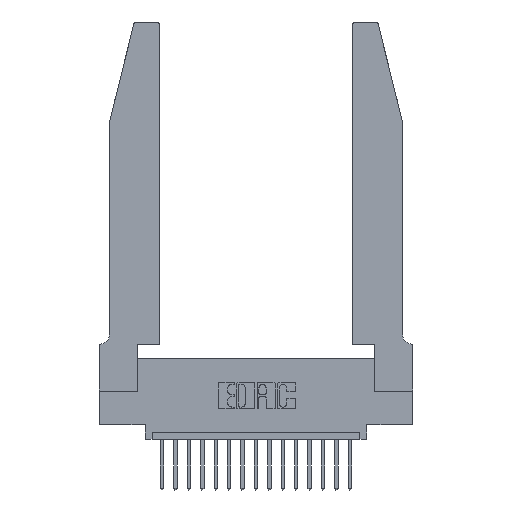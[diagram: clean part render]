
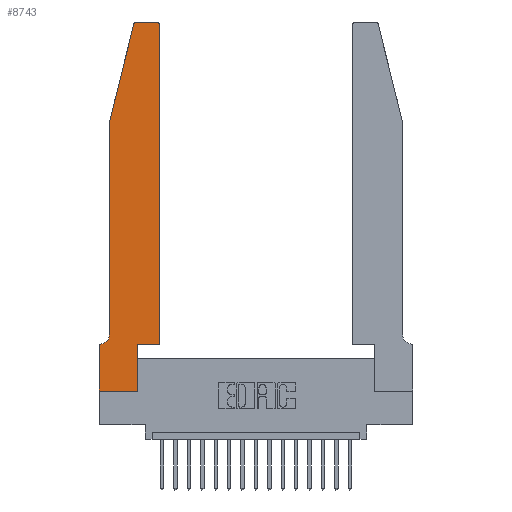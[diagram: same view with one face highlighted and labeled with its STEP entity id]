
A CAD part, top view. The second image highlights one B-rep face of the part: STEP entity #8743.
In plain terms, the highlighted planar face has unit normal (0, 0, 1).
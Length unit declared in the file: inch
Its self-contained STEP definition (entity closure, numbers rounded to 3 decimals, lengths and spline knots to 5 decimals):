
#88 = VECTOR ( 'NONE', #19407, 39.37008 ) ;
#260 = CIRCLE ( 'NONE', #11740, 0.03 ) ;
#834 = VERTEX_POINT ( 'NONE', #14219 ) ;
#893 = CIRCLE ( 'NONE', #18518, 0.03 ) ;
#983 = ORIENTED_EDGE ( 'NONE', *, *, #5429, .T. ) ;
#1018 = VECTOR ( 'NONE', #5534, 39.37008 ) ;
#1057 = FACE_OUTER_BOUND ( 'NONE', #17933, .T. ) ;
#1080 = VERTEX_POINT ( 'NONE', #16287 ) ;
#1220 = CARTESIAN_POINT ( 'NONE',  ( 0.0055, 0.42, 0.37 ) ) ;
#1270 = DIRECTION ( 'NONE',  ( 0., 1., 0. ) ) ;
#1604 = VERTEX_POINT ( 'NONE', #9121 ) ;
#2000 = EDGE_CURVE ( 'NONE', #5994, #1080, #260, .T. ) ;
#2140 = CARTESIAN_POINT ( 'NONE',  ( 0.25487, 2.72718, 0.37 ) ) ;
#2611 = LINE ( 'NONE', #16201, #7883 ) ;
#3807 = ORIENTED_EDGE ( 'NONE', *, *, #18203, .T. ) ;
#3827 = ORIENTED_EDGE ( 'NONE', *, *, #16820, .T. ) ;
#3977 = VERTEX_POINT ( 'NONE', #17043 ) ;
#4001 = VERTEX_POINT ( 'NONE', #5031 ) ;
#4025 = DIRECTION ( 'NONE',  ( 1., 0., 0. ) ) ;
#4074 = VERTEX_POINT ( 'NONE', #11245 ) ;
#4116 = LINE ( 'NONE', #8658, #88 ) ;
#4330 = LINE ( 'NONE', #9478, #1018 ) ;
#4439 = DIRECTION ( 'NONE',  ( -1., 0., 0. ) ) ;
#4830 = VERTEX_POINT ( 'NONE', #12099 ) ;
#5031 = CARTESIAN_POINT ( 'NONE',  ( 0.0055, 0.35, 0.37 ) ) ;
#5297 = VECTOR ( 'NONE', #4439, 39.37008 ) ;
#5429 = EDGE_CURVE ( 'NONE', #4074, #5994, #6590, .T. ) ;
#5534 = DIRECTION ( 'NONE',  ( 1., 0., 0. ) ) ;
#5660 = DIRECTION ( 'NONE',  ( -1., 0., 0. ) ) ;
#5920 = VECTOR ( 'NONE', #12808, 39.37008 ) ;
#5974 = EDGE_CURVE ( 'NONE', #13099, #4001, #12536, .T. ) ;
#5994 = VERTEX_POINT ( 'NONE', #8876 ) ;
#6364 = CARTESIAN_POINT ( 'NONE',  ( 0., 0., 0.37 ) ) ;
#6590 = LINE ( 'NONE', #9124, #18580 ) ;
#6973 = PLANE ( 'NONE',  #10101 ) ;
#7408 = VECTOR ( 'NONE', #11637, 39.37008 ) ;
#7510 = ORIENTED_EDGE ( 'NONE', *, *, #14543, .T. ) ;
#7883 = VECTOR ( 'NONE', #5660, 39.37008 ) ;
#7919 = CARTESIAN_POINT ( 'NONE',  ( 0.284, 2.72, 0.37 ) ) ;
#8313 = ORIENTED_EDGE ( 'NONE', *, *, #17639, .T. ) ;
#8387 = CARTESIAN_POINT ( 'NONE',  ( 0., 0.35, 0.37 ) ) ;
#8507 = DIRECTION ( 'NONE',  ( 0., 0., 1. ) ) ;
#8658 = CARTESIAN_POINT ( 'NONE',  ( 0.0755, 2., 0.37 ) ) ;
#8666 = CARTESIAN_POINT ( 'NONE',  ( 0.4505, 0.35, 0.37 ) ) ;
#8684 = VERTEX_POINT ( 'NONE', #2140 ) ;
#8743 = ADVANCED_FACE ( 'NONE', ( #1057 ), #6973, .T. ) ;
#8761 = LINE ( 'NONE', #11251, #5920 ) ;
#8876 = CARTESIAN_POINT ( 'NONE',  ( 0.4505, 2.72, 0.37 ) ) ;
#9121 = CARTESIAN_POINT ( 'NONE',  ( 0.2865, 0.35, 0.37 ) ) ;
#9124 = CARTESIAN_POINT ( 'NONE',  ( 0.4505, 0.35, 0.37 ) ) ;
#9411 = EDGE_CURVE ( 'NONE', #8684, #18680, #4116, .T. ) ;
#9478 = CARTESIAN_POINT ( 'NONE',  ( 0., 0., 0.37 ) ) ;
#9704 = LINE ( 'NONE', #6364, #10393 ) ;
#10101 = AXIS2_PLACEMENT_3D ( 'NONE', #8387, #8507, #17453 ) ;
#10141 = VERTEX_POINT ( 'NONE', #14768 ) ;
#10278 = AXIS2_PLACEMENT_3D ( 'NONE', #1220, #18346, #15186 ) ;
#10393 = VECTOR ( 'NONE', #18820, 39.37008 ) ;
#10521 = CARTESIAN_POINT ( 'NONE',  ( 0.0755, 0.35, 0.37 ) ) ;
#10523 = LINE ( 'NONE', #10521, #5297 ) ;
#10629 = CARTESIAN_POINT ( 'NONE',  ( 0.0755, 0.42, 0.37 ) ) ;
#11245 = CARTESIAN_POINT ( 'NONE',  ( 0.4505, 0.35, 0.37 ) ) ;
#11251 = CARTESIAN_POINT ( 'NONE',  ( 0.0755, 2., 0.37 ) ) ;
#11637 = DIRECTION ( 'NONE',  ( 0., 1., 0. ) ) ;
#11698 = CARTESIAN_POINT ( 'NONE',  ( 0.4205, 2.72, 0.37 ) ) ;
#11740 = AXIS2_PLACEMENT_3D ( 'NONE', #11698, #17776, #4025 ) ;
#12099 = CARTESIAN_POINT ( 'NONE',  ( 0.284, 2.75, 0.37 ) ) ;
#12390 = ORIENTED_EDGE ( 'NONE', *, *, #17186, .T. ) ;
#12536 = CIRCLE ( 'NONE', #10278, 0.07 ) ;
#12636 = ORIENTED_EDGE ( 'NONE', *, *, #9411, .T. ) ;
#12808 = DIRECTION ( 'NONE',  ( 0., -1., 0. ) ) ;
#13099 = VERTEX_POINT ( 'NONE', #10629 ) ;
#13935 = EDGE_CURVE ( 'NONE', #4830, #8684, #893, .T. ) ;
#14219 = CARTESIAN_POINT ( 'NONE',  ( 0., 0.35, 0.37 ) ) ;
#14221 = EDGE_CURVE ( 'NONE', #834, #3977, #9704, .T. ) ;
#14241 = ORIENTED_EDGE ( 'NONE', *, *, #19699, .T. ) ;
#14543 = EDGE_CURVE ( 'NONE', #1604, #4074, #17262, .T. ) ;
#14768 = CARTESIAN_POINT ( 'NONE',  ( 0.2865, 0., 0.37 ) ) ;
#15088 = ORIENTED_EDGE ( 'NONE', *, *, #2000, .T. ) ;
#15186 = DIRECTION ( 'NONE',  ( -1., 0., 0. ) ) ;
#15742 = ORIENTED_EDGE ( 'NONE', *, *, #13935, .T. ) ;
#16014 = ORIENTED_EDGE ( 'NONE', *, *, #14221, .T. ) ;
#16035 = VECTOR ( 'NONE', #19416, 39.37008 ) ;
#16201 = CARTESIAN_POINT ( 'NONE',  ( 0.2605, 2.75, 0.37 ) ) ;
#16287 = CARTESIAN_POINT ( 'NONE',  ( 0.4205, 2.75, 0.37 ) ) ;
#16594 = DIRECTION ( 'NONE',  ( 0., 0., 1. ) ) ;
#16786 = LINE ( 'NONE', #17595, #7408 ) ;
#16820 = EDGE_CURVE ( 'NONE', #3977, #10141, #4330, .T. ) ;
#17043 = CARTESIAN_POINT ( 'NONE',  ( 0., 0., 0.37 ) ) ;
#17186 = EDGE_CURVE ( 'NONE', #4001, #834, #10523, .T. ) ;
#17262 = LINE ( 'NONE', #8666, #16035 ) ;
#17345 = ORIENTED_EDGE ( 'NONE', *, *, #5974, .T. ) ;
#17453 = DIRECTION ( 'NONE',  ( 1., 0., 0. ) ) ;
#17595 = CARTESIAN_POINT ( 'NONE',  ( 0.2865, 0.35, 0.37 ) ) ;
#17639 = EDGE_CURVE ( 'NONE', #10141, #1604, #16786, .T. ) ;
#17668 = CARTESIAN_POINT ( 'NONE',  ( 0.0755, 2., 0.37 ) ) ;
#17776 = DIRECTION ( 'NONE',  ( 0., 0., 1. ) ) ;
#17933 = EDGE_LOOP ( 'NONE', ( #3807, #15742, #12636, #14241, #17345, #12390, #16014, #3827, #8313, #7510, #983, #15088 ) ) ;
#18149 = DIRECTION ( 'NONE',  ( 1., 0., 0. ) ) ;
#18203 = EDGE_CURVE ( 'NONE', #1080, #4830, #2611, .T. ) ;
#18346 = DIRECTION ( 'NONE',  ( 0., 0., -1. ) ) ;
#18518 = AXIS2_PLACEMENT_3D ( 'NONE', #7919, #16594, #18149 ) ;
#18580 = VECTOR ( 'NONE', #1270, 39.37008 ) ;
#18680 = VERTEX_POINT ( 'NONE', #17668 ) ;
#18820 = DIRECTION ( 'NONE',  ( 0., -1., 0. ) ) ;
#19407 = DIRECTION ( 'NONE',  ( -0.239, -0.971, 0. ) ) ;
#19416 = DIRECTION ( 'NONE',  ( 1., 0., 0. ) ) ;
#19699 = EDGE_CURVE ( 'NONE', #18680, #13099, #8761, .T. ) ;
